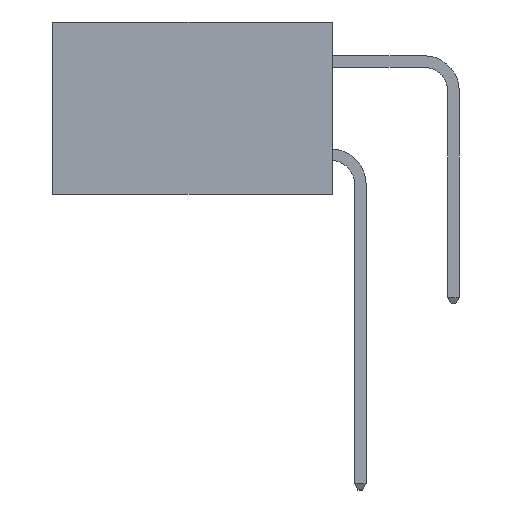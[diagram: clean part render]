
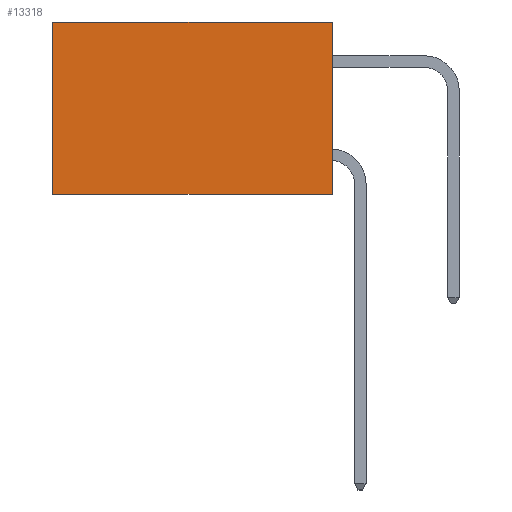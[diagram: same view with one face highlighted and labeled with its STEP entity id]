
A CAD part, left-side view. The second image highlights one B-rep face of the part: STEP entity #13318.
In plain terms, the highlighted planar face has unit normal (-1, 0, 0).
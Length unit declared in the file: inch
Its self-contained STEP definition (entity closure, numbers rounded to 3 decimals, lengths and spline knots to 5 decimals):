
#48 = CARTESIAN_POINT ( 'NONE',  ( 0.2615, 0.6, -0.37 ) ) ;
#426 = PLANE ( 'NONE',  #5731 ) ;
#1574 = ORIENTED_EDGE ( 'NONE', *, *, #3810, .T. ) ;
#1630 = EDGE_CURVE ( 'NONE', #13669, #1895, #9883, .T. ) ;
#1895 = VERTEX_POINT ( 'NONE', #12132 ) ;
#2014 = ORIENTED_EDGE ( 'NONE', *, *, #7119, .F. ) ;
#3199 = DIRECTION ( 'NONE',  ( 1., 0., 0. ) ) ;
#3810 = EDGE_CURVE ( 'NONE', #1895, #8265, #6901, .T. ) ;
#3851 = CARTESIAN_POINT ( 'NONE',  ( 0.2615, 0., -0.37 ) ) ;
#3945 = VECTOR ( 'NONE', #11154, 39.37008 ) ;
#4640 = DIRECTION ( 'NONE',  ( 0., 1., 0. ) ) ;
#5437 = CARTESIAN_POINT ( 'NONE',  ( 0.2615, 0., 0. ) ) ;
#5467 = DIRECTION ( 'NONE',  ( 0., 1., 0. ) ) ;
#5731 = AXIS2_PLACEMENT_3D ( 'NONE', #6935, #3199, #11915 ) ;
#6581 = VERTEX_POINT ( 'NONE', #16100 ) ;
#6901 = LINE ( 'NONE', #11341, #3945 ) ;
#6935 = CARTESIAN_POINT ( 'NONE',  ( 0.2615, 0., -0.37 ) ) ;
#7119 = EDGE_CURVE ( 'NONE', #13669, #6581, #13539, .T. ) ;
#8265 = VERTEX_POINT ( 'NONE', #48 ) ;
#8355 = ORIENTED_EDGE ( 'NONE', *, *, #11284, .F. ) ;
#8763 = ORIENTED_EDGE ( 'NONE', *, *, #1630, .T. ) ;
#9857 = VECTOR ( 'NONE', #14322, 39.37008 ) ;
#9883 = LINE ( 'NONE', #5437, #15909 ) ;
#11154 = DIRECTION ( 'NONE',  ( 0., 0., -1. ) ) ;
#11284 = EDGE_CURVE ( 'NONE', #6581, #8265, #15304, .T. ) ;
#11329 = CARTESIAN_POINT ( 'NONE',  ( 0.2615, 0., 0. ) ) ;
#11341 = CARTESIAN_POINT ( 'NONE',  ( 0.2615, 0.6, -0.37 ) ) ;
#11915 = DIRECTION ( 'NONE',  ( 0., 0., -1. ) ) ;
#12106 = VECTOR ( 'NONE', #4640, 39.37008 ) ;
#12132 = CARTESIAN_POINT ( 'NONE',  ( 0.2615, 0.6, 0. ) ) ;
#13318 = ADVANCED_FACE ( 'NONE', ( #14228 ), #426, .F. ) ;
#13539 = LINE ( 'NONE', #14372, #9857 ) ;
#13669 = VERTEX_POINT ( 'NONE', #11329 ) ;
#14228 = FACE_OUTER_BOUND ( 'NONE', #15563, .T. ) ;
#14322 = DIRECTION ( 'NONE',  ( 0., 0., -1. ) ) ;
#14372 = CARTESIAN_POINT ( 'NONE',  ( 0.2615, 0., -0.37 ) ) ;
#15304 = LINE ( 'NONE', #3851, #12106 ) ;
#15563 = EDGE_LOOP ( 'NONE', ( #1574, #8355, #2014, #8763 ) ) ;
#15909 = VECTOR ( 'NONE', #5467, 39.37008 ) ;
#16100 = CARTESIAN_POINT ( 'NONE',  ( 0.2615, 0., -0.37 ) ) ;
